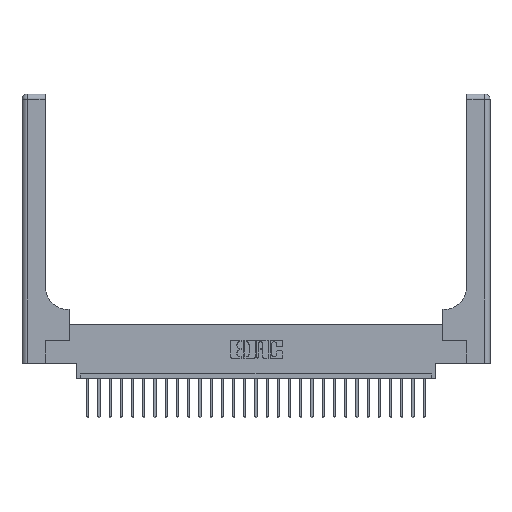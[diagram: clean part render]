
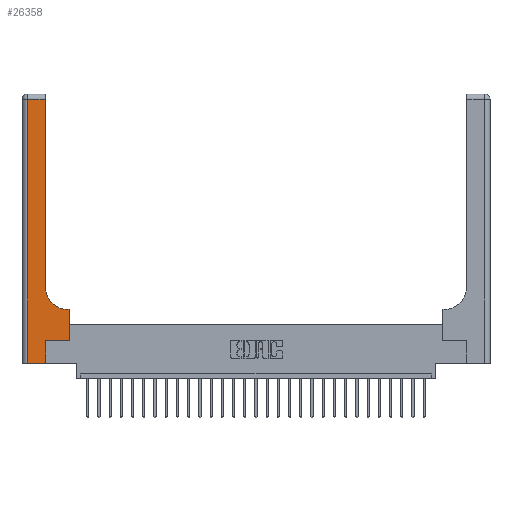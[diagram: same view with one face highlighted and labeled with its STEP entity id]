
A CAD part, top view. The second image highlights one B-rep face of the part: STEP entity #26358.
In plain terms, the highlighted planar face has unit normal (0, 0, 1).
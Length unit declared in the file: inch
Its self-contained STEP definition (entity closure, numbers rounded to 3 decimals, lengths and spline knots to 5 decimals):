
#249 = VECTOR ( 'NONE', #16801, 39.37008 ) ;
#407 = VERTEX_POINT ( 'NONE', #3437 ) ;
#1197 = DIRECTION ( 'NONE',  ( 1., 0., 0. ) ) ;
#1265 = VECTOR ( 'NONE', #11915, 39.37008 ) ;
#2069 = LINE ( 'NONE', #11957, #18690 ) ;
#2402 = CARTESIAN_POINT ( 'NONE',  ( 0.06, 2.94, 0.37 ) ) ;
#2740 = DIRECTION ( 'NONE',  ( 0., 1., 0. ) ) ;
#2817 = VECTOR ( 'NONE', #1197, 39.37008 ) ;
#2934 = LINE ( 'NONE', #23714, #2817 ) ;
#3322 = CARTESIAN_POINT ( 'NONE',  ( 0.26, 0.85, 0.37 ) ) ;
#3437 = CARTESIAN_POINT ( 'NONE',  ( 0.528, 0.25, 0.37 ) ) ;
#4734 = ORIENTED_EDGE ( 'NONE', *, *, #9233, .T. ) ;
#5049 = ORIENTED_EDGE ( 'NONE', *, *, #25956, .T. ) ;
#5673 = DIRECTION ( 'NONE',  ( -1., 0., 0. ) ) ;
#5931 = PLANE ( 'NONE',  #6666 ) ;
#6543 = LINE ( 'NONE', #18864, #9463 ) ;
#6666 = AXIS2_PLACEMENT_3D ( 'NONE', #15840, #24048, #5673 ) ;
#7511 = LINE ( 'NONE', #25769, #8517 ) ;
#7848 = DIRECTION ( 'NONE',  ( 0., 1., 0. ) ) ;
#7978 = VERTEX_POINT ( 'NONE', #20162 ) ;
#8146 = CARTESIAN_POINT ( 'NONE',  ( 0.265, 0., 0.37 ) ) ;
#8467 = VERTEX_POINT ( 'NONE', #2402 ) ;
#8517 = VECTOR ( 'NONE', #9529, 39.37008 ) ;
#8702 = VERTEX_POINT ( 'NONE', #3322 ) ;
#8707 = EDGE_LOOP ( 'NONE', ( #18487, #19842, #4734, #23999, #5049, #10128, #12410, #18896, #19165 ) ) ;
#9233 = EDGE_CURVE ( 'NONE', #8467, #7978, #2069, .T. ) ;
#9463 = VECTOR ( 'NONE', #15620, 39.37008 ) ;
#9529 = DIRECTION ( 'NONE',  ( -1., 0., 0. ) ) ;
#10128 = ORIENTED_EDGE ( 'NONE', *, *, #24117, .T. ) ;
#11553 = CARTESIAN_POINT ( 'NONE',  ( 0.265, 0.25, 0.37 ) ) ;
#11739 = EDGE_CURVE ( 'NONE', #15272, #14014, #7511, .T. ) ;
#11915 = DIRECTION ( 'NONE',  ( -1., 0., 0. ) ) ;
#11957 = CARTESIAN_POINT ( 'NONE',  ( 0.06, 3., 0.37 ) ) ;
#12070 = VERTEX_POINT ( 'NONE', #19161 ) ;
#12356 = VERTEX_POINT ( 'NONE', #8146 ) ;
#12410 = ORIENTED_EDGE ( 'NONE', *, *, #14602, .T. ) ;
#12495 = EDGE_CURVE ( 'NONE', #7978, #12356, #6543, .T. ) ;
#12592 = DIRECTION ( 'NONE',  ( 0., 0., -1. ) ) ;
#12620 = CIRCLE ( 'NONE', #14783, 0.25 ) ;
#13876 = EDGE_CURVE ( 'NONE', #8702, #12070, #17904, .T. ) ;
#14014 = VERTEX_POINT ( 'NONE', #22206 ) ;
#14084 = FACE_OUTER_BOUND ( 'NONE', #8707, .T. ) ;
#14118 = LINE ( 'NONE', #22327, #249 ) ;
#14602 = EDGE_CURVE ( 'NONE', #407, #15272, #21088, .T. ) ;
#14783 = AXIS2_PLACEMENT_3D ( 'NONE', #20414, #12592, #22953 ) ;
#15158 = CARTESIAN_POINT ( 'NONE',  ( 0.528, 0.25, 0.37 ) ) ;
#15272 = VERTEX_POINT ( 'NONE', #20415 ) ;
#15620 = DIRECTION ( 'NONE',  ( 1., 0., 0. ) ) ;
#15840 = CARTESIAN_POINT ( 'NONE',  ( 0., 3., 0.37 ) ) ;
#15865 = VECTOR ( 'NONE', #7848, 39.37008 ) ;
#16801 = DIRECTION ( 'NONE',  ( 0., 1., 0. ) ) ;
#16882 = EDGE_CURVE ( 'NONE', #12070, #8467, #24021, .T. ) ;
#17904 = LINE ( 'NONE', #25704, #15865 ) ;
#18487 = ORIENTED_EDGE ( 'NONE', *, *, #13876, .T. ) ;
#18690 = VECTOR ( 'NONE', #24185, 39.37008 ) ;
#18864 = CARTESIAN_POINT ( 'NONE',  ( 0., 0., 0.37 ) ) ;
#18896 = ORIENTED_EDGE ( 'NONE', *, *, #11739, .T. ) ;
#19161 = CARTESIAN_POINT ( 'NONE',  ( 0.26, 2.94, 0.37 ) ) ;
#19165 = ORIENTED_EDGE ( 'NONE', *, *, #26480, .T. ) ;
#19842 = ORIENTED_EDGE ( 'NONE', *, *, #16882, .T. ) ;
#19865 = CARTESIAN_POINT ( 'NONE',  ( 0., 2.94, 0.37 ) ) ;
#20162 = CARTESIAN_POINT ( 'NONE',  ( 0.06, 0., 0.37 ) ) ;
#20414 = CARTESIAN_POINT ( 'NONE',  ( 0.51, 0.85, 0.37 ) ) ;
#20415 = CARTESIAN_POINT ( 'NONE',  ( 0.528, 0.6, 0.37 ) ) ;
#20965 = VERTEX_POINT ( 'NONE', #11553 ) ;
#21088 = LINE ( 'NONE', #15158, #21562 ) ;
#21562 = VECTOR ( 'NONE', #2740, 39.37008 ) ;
#22206 = CARTESIAN_POINT ( 'NONE',  ( 0.51, 0.6, 0.37 ) ) ;
#22327 = CARTESIAN_POINT ( 'NONE',  ( 0.265, 0., 0.37 ) ) ;
#22953 = DIRECTION ( 'NONE',  ( 1., 0., 0. ) ) ;
#23714 = CARTESIAN_POINT ( 'NONE',  ( 0.265, 0.25, 0.37 ) ) ;
#23999 = ORIENTED_EDGE ( 'NONE', *, *, #12495, .T. ) ;
#24021 = LINE ( 'NONE', #19865, #1265 ) ;
#24048 = DIRECTION ( 'NONE',  ( 0., 0., -1. ) ) ;
#24117 = EDGE_CURVE ( 'NONE', #20965, #407, #2934, .T. ) ;
#24185 = DIRECTION ( 'NONE',  ( 0., -1., 0. ) ) ;
#25704 = CARTESIAN_POINT ( 'NONE',  ( 0.26, 3., 0.37 ) ) ;
#25769 = CARTESIAN_POINT ( 'NONE',  ( 0.26, 0.6, 0.37 ) ) ;
#25956 = EDGE_CURVE ( 'NONE', #12356, #20965, #14118, .T. ) ;
#26358 = ADVANCED_FACE ( 'NONE', ( #14084 ), #5931, .F. ) ;
#26480 = EDGE_CURVE ( 'NONE', #14014, #8702, #12620, .T. ) ;
